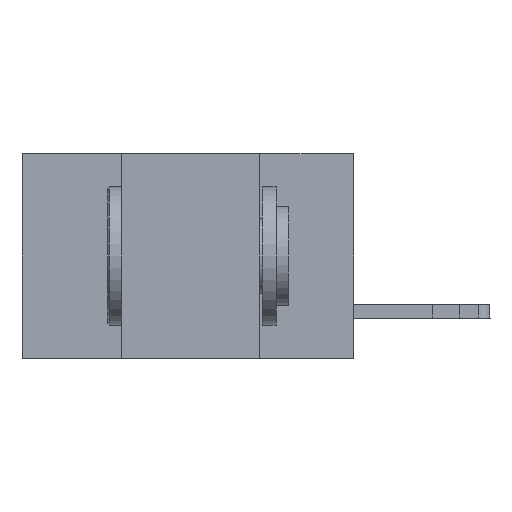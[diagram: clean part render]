
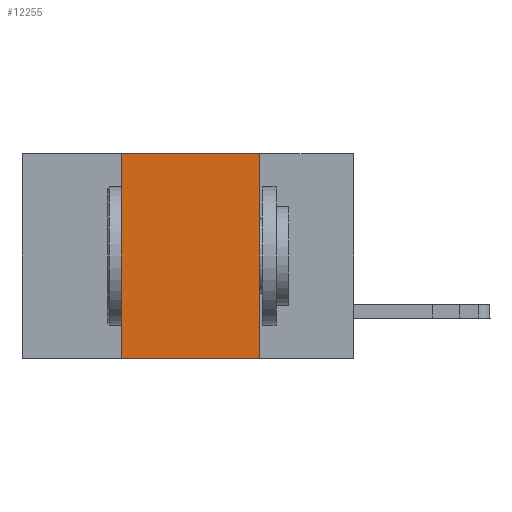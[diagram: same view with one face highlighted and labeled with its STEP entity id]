
A CAD part, left-side view. The second image highlights one B-rep face of the part: STEP entity #12255.
In plain terms, the highlighted planar face has unit normal (-1, 0, 0).
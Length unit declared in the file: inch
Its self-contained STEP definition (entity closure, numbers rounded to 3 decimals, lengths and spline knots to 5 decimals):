
#573 = DIRECTION ( 'NONE',  ( 0., 0., 1. ) ) ;
#1836 = DIRECTION ( 'NONE',  ( 0., 0., -1. ) ) ;
#3217 = VERTEX_POINT ( 'NONE', #5219 ) ;
#3219 = DIRECTION ( 'NONE',  ( 0., -1., 0. ) ) ;
#3340 = CARTESIAN_POINT ( 'NONE',  ( 0., 0.6, 0. ) ) ;
#3360 = CARTESIAN_POINT ( 'NONE',  ( 0., 0.6, -0.37 ) ) ;
#4751 = ORIENTED_EDGE ( 'NONE', *, *, #6956, .F. ) ;
#4840 = PLANE ( 'NONE',  #24893 ) ;
#4944 = CARTESIAN_POINT ( 'NONE',  ( 0., 0.17, 0. ) ) ;
#5094 = CARTESIAN_POINT ( 'NONE',  ( 0., 0.42, 0. ) ) ;
#5219 = CARTESIAN_POINT ( 'NONE',  ( 0., 0.17, 0. ) ) ;
#5867 = DIRECTION ( 'NONE',  ( 0., -1., 0. ) ) ;
#6956 = EDGE_CURVE ( 'NONE', #3217, #16109, #7568, .T. ) ;
#7568 = LINE ( 'NONE', #4944, #17711 ) ;
#8571 = CARTESIAN_POINT ( 'NONE',  ( 0., 0.42, 0. ) ) ;
#9430 = ORIENTED_EDGE ( 'NONE', *, *, #26122, .F. ) ;
#12255 = ADVANCED_FACE ( 'NONE', ( #31045 ), #4840, .F. ) ;
#16012 = LINE ( 'NONE', #3340, #19574 ) ;
#16060 = DIRECTION ( 'NONE',  ( 1., 0., 0. ) ) ;
#16109 = VERTEX_POINT ( 'NONE', #21286 ) ;
#16378 = VERTEX_POINT ( 'NONE', #26374 ) ;
#17187 = VECTOR ( 'NONE', #5867, 39.37008 ) ;
#17711 = VECTOR ( 'NONE', #1836, 39.37008 ) ;
#17795 = EDGE_CURVE ( 'NONE', #28176, #3217, #16012, .T. ) ;
#19574 = VECTOR ( 'NONE', #3219, 39.37008 ) ;
#21258 = EDGE_CURVE ( 'NONE', #16378, #16109, #31343, .T. ) ;
#21286 = CARTESIAN_POINT ( 'NONE',  ( 0., 0.17, -0.37 ) ) ;
#24893 = AXIS2_PLACEMENT_3D ( 'NONE', #27248, #16060, #27495 ) ;
#26122 = EDGE_CURVE ( 'NONE', #16378, #28176, #29767, .T. ) ;
#26374 = CARTESIAN_POINT ( 'NONE',  ( 0., 0.42, -0.37 ) ) ;
#27248 = CARTESIAN_POINT ( 'NONE',  ( 0., 0.6, 0. ) ) ;
#27495 = DIRECTION ( 'NONE',  ( 0., 0., -1. ) ) ;
#28176 = VERTEX_POINT ( 'NONE', #8571 ) ;
#29767 = LINE ( 'NONE', #5094, #30228 ) ;
#30228 = VECTOR ( 'NONE', #573, 39.37008 ) ;
#31045 = FACE_OUTER_BOUND ( 'NONE', #36588, .T. ) ;
#31343 = LINE ( 'NONE', #3360, #17187 ) ;
#31811 = ORIENTED_EDGE ( 'NONE', *, *, #17795, .F. ) ;
#34718 = ORIENTED_EDGE ( 'NONE', *, *, #21258, .T. ) ;
#36588 = EDGE_LOOP ( 'NONE', ( #4751, #31811, #9430, #34718 ) ) ;
